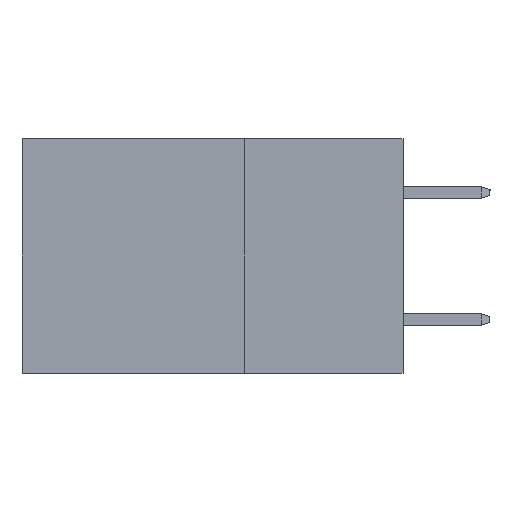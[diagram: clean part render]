
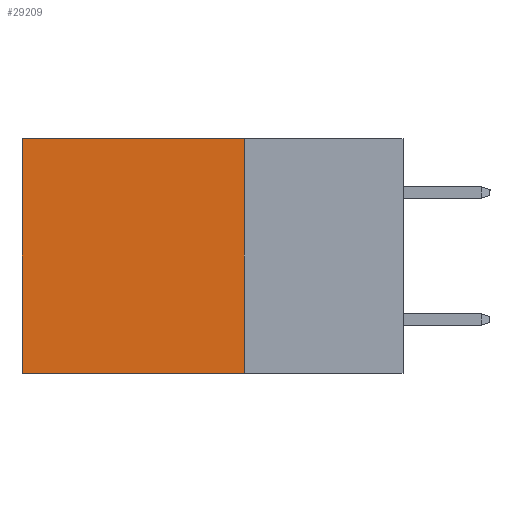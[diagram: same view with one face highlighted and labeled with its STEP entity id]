
A CAD part, left-side view. The second image highlights one B-rep face of the part: STEP entity #29209.
In plain terms, the highlighted planar face has unit normal (-1, 0, 0).
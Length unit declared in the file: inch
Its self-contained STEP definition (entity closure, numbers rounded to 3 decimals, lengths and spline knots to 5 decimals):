
#3284 = CARTESIAN_POINT ( 'NONE',  ( 0.2875, 0.6, 0. ) ) ;
#3833 = EDGE_LOOP ( 'NONE', ( #28956, #4143, #12157, #4105 ) ) ;
#4105 = ORIENTED_EDGE ( 'NONE', *, *, #22973, .T. ) ;
#4143 = ORIENTED_EDGE ( 'NONE', *, *, #17800, .F. ) ;
#4686 = CARTESIAN_POINT ( 'NONE',  ( 0.2875, 0.25, 0. ) ) ;
#5520 = LINE ( 'NONE', #3284, #30195 ) ;
#5632 = CARTESIAN_POINT ( 'NONE',  ( 0.2875, 0.25, 0. ) ) ;
#8199 = LINE ( 'NONE', #5632, #32251 ) ;
#8390 = VECTOR ( 'NONE', #9031, 39.37008 ) ;
#9031 = DIRECTION ( 'NONE',  ( 0., 1., 0. ) ) ;
#10220 = VERTEX_POINT ( 'NONE', #12116 ) ;
#10620 = EDGE_CURVE ( 'NONE', #23455, #10220, #8199, .T. ) ;
#10685 = FACE_OUTER_BOUND ( 'NONE', #3833, .T. ) ;
#11355 = CARTESIAN_POINT ( 'NONE',  ( 0.2875, 0.25, 0. ) ) ;
#12116 = CARTESIAN_POINT ( 'NONE',  ( 0.2875, 0.25, -0.37 ) ) ;
#12157 = ORIENTED_EDGE ( 'NONE', *, *, #10620, .F. ) ;
#13255 = DIRECTION ( 'NONE',  ( 1., 0., 0. ) ) ;
#13997 = VECTOR ( 'NONE', #33340, 39.37008 ) ;
#14461 = VERTEX_POINT ( 'NONE', #30118 ) ;
#15917 = DIRECTION ( 'NONE',  ( 0., 0., -1. ) ) ;
#16060 = EDGE_CURVE ( 'NONE', #19864, #14461, #5520, .T. ) ;
#17800 = EDGE_CURVE ( 'NONE', #10220, #14461, #30025, .T. ) ;
#19864 = VERTEX_POINT ( 'NONE', #25297 ) ;
#19924 = CARTESIAN_POINT ( 'NONE',  ( 0.2875, 0.25, -0.37 ) ) ;
#21781 = DIRECTION ( 'NONE',  ( 0., 0., -1. ) ) ;
#22973 = EDGE_CURVE ( 'NONE', #23455, #19864, #33161, .T. ) ;
#23455 = VERTEX_POINT ( 'NONE', #31252 ) ;
#24337 = PLANE ( 'NONE',  #28933 ) ;
#25297 = CARTESIAN_POINT ( 'NONE',  ( 0.2875, 0.6, 0. ) ) ;
#26424 = DIRECTION ( 'NONE',  ( 0., 0., -1. ) ) ;
#28933 = AXIS2_PLACEMENT_3D ( 'NONE', #11355, #13255, #21781 ) ;
#28956 = ORIENTED_EDGE ( 'NONE', *, *, #16060, .T. ) ;
#29209 = ADVANCED_FACE ( 'NONE', ( #10685 ), #24337, .F. ) ;
#30025 = LINE ( 'NONE', #19924, #8390 ) ;
#30118 = CARTESIAN_POINT ( 'NONE',  ( 0.2875, 0.6, -0.37 ) ) ;
#30195 = VECTOR ( 'NONE', #15917, 39.37008 ) ;
#31252 = CARTESIAN_POINT ( 'NONE',  ( 0.2875, 0.25, 0. ) ) ;
#32251 = VECTOR ( 'NONE', #26424, 39.37008 ) ;
#33161 = LINE ( 'NONE', #4686, #13997 ) ;
#33340 = DIRECTION ( 'NONE',  ( 0., 1., 0. ) ) ;
